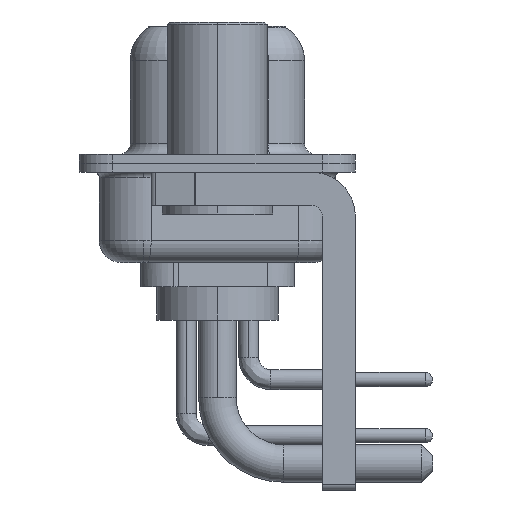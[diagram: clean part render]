
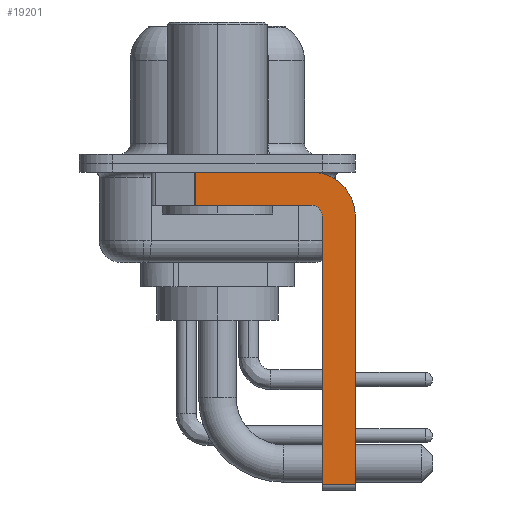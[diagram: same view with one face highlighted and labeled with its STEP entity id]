
A CAD part, left-side view. The second image highlights one B-rep face of the part: STEP entity #19201.
In plain terms, the highlighted planar face has unit normal (-1, 0, 0).
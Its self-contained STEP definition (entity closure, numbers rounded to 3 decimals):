
#447 = ORIENTED_EDGE ( 'NONE', *, *, #19779, .F. ) ;
#1129 = ORIENTED_EDGE ( 'NONE', *, *, #11732, .F. ) ;
#1615 = VERTEX_POINT ( 'NONE', #15081 ) ;
#2427 = CARTESIAN_POINT ( 'NONE',  ( -2.9, -6.25, -2.4 ) ) ;
#2546 = ORIENTED_EDGE ( 'NONE', *, *, #19174, .F. ) ;
#2817 = VERTEX_POINT ( 'NONE', #10769 ) ;
#2862 = CARTESIAN_POINT ( 'NONE',  ( -2.9, -4.25, -2.4 ) ) ;
#3093 = LINE ( 'NONE', #10649, #10733 ) ;
#3225 = DIRECTION ( 'NONE',  ( -1., 0., 0. ) ) ;
#3245 = CARTESIAN_POINT ( 'NONE',  ( -2.9, -6.25, -14.55 ) ) ;
#3899 = LINE ( 'NONE', #17183, #10660 ) ;
#4095 = LINE ( 'NONE', #12005, #23969 ) ;
#4127 = AXIS2_PLACEMENT_3D ( 'NONE', #22752, #5484, #19265 ) ;
#4213 = DIRECTION ( 'NONE',  ( 0., 0., 1. ) ) ;
#4523 = CARTESIAN_POINT ( 'NONE',  ( -2.9, -4.25, -0.4 ) ) ;
#4840 = ORIENTED_EDGE ( 'NONE', *, *, #5111, .F. ) ;
#4882 = ORIENTED_EDGE ( 'NONE', *, *, #15754, .T. ) ;
#5111 = EDGE_CURVE ( 'NONE', #7124, #20126, #13073, .T. ) ;
#5203 = CARTESIAN_POINT ( 'NONE',  ( -2.9, -4.25, -1.9 ) ) ;
#5484 = DIRECTION ( 'NONE',  ( 1., 0., 0. ) ) ;
#5580 = LINE ( 'NONE', #5203, #17742 ) ;
#6432 = EDGE_CURVE ( 'NONE', #2817, #1615, #10281, .T. ) ;
#6849 = ORIENTED_EDGE ( 'NONE', *, *, #19059, .T. ) ;
#7124 = VERTEX_POINT ( 'NONE', #4523 ) ;
#7460 = DIRECTION ( 'NONE',  ( 0., 0., -1. ) ) ;
#7976 = ORIENTED_EDGE ( 'NONE', *, *, #6432, .F. ) ;
#9322 = CARTESIAN_POINT ( 'NONE',  ( -2.9, -6.25, -2.4 ) ) ;
#9692 = LINE ( 'NONE', #9322, #15206 ) ;
#9951 = CARTESIAN_POINT ( 'NONE',  ( -2.9, -4.75, -14.55 ) ) ;
#10281 = CIRCLE ( 'NONE', #20623, 0.5 ) ;
#10412 = DIRECTION ( 'NONE',  ( 0., 0., 1. ) ) ;
#10649 = CARTESIAN_POINT ( 'NONE',  ( -2.9, 3., -0.4 ) ) ;
#10660 = VECTOR ( 'NONE', #15302, 1000. ) ;
#10733 = VECTOR ( 'NONE', #11259, 1000. ) ;
#10769 = CARTESIAN_POINT ( 'NONE',  ( -2.9, -4.75, -2.4 ) ) ;
#11234 = VERTEX_POINT ( 'NONE', #3245 ) ;
#11259 = DIRECTION ( 'NONE',  ( 0., -1., 0. ) ) ;
#11595 = VERTEX_POINT ( 'NONE', #14501 ) ;
#11732 = EDGE_CURVE ( 'NONE', #1615, #11595, #5580, .T. ) ;
#12005 = CARTESIAN_POINT ( 'NONE',  ( -2.9, -4.75, -14.8 ) ) ;
#12376 = CARTESIAN_POINT ( 'NONE',  ( -2.9, -4.25, -2.4 ) ) ;
#12495 = DIRECTION ( 'NONE',  ( 1., 0., 0. ) ) ;
#12826 = VECTOR ( 'NONE', #18406, 1000. ) ;
#12889 = DIRECTION ( 'NONE',  ( 0., 1., 0. ) ) ;
#13073 = CIRCLE ( 'NONE', #18640, 2. ) ;
#14042 = VERTEX_POINT ( 'NONE', #18023 ) ;
#14471 = EDGE_LOOP ( 'NONE', ( #15629, #4882, #1129, #7976, #447, #6849, #2546, #4840 ) ) ;
#14501 = CARTESIAN_POINT ( 'NONE',  ( -2.9, 0.978, -1.9 ) ) ;
#14803 = EDGE_CURVE ( 'NONE', #14042, #7124, #3093, .T. ) ;
#15081 = CARTESIAN_POINT ( 'NONE',  ( -2.9, -4.25, -1.9 ) ) ;
#15206 = VECTOR ( 'NONE', #7460, 1000. ) ;
#15302 = DIRECTION ( 'NONE',  ( 0., 0., -1. ) ) ;
#15629 = ORIENTED_EDGE ( 'NONE', *, *, #14803, .F. ) ;
#15754 = EDGE_CURVE ( 'NONE', #14042, #11595, #3899, .T. ) ;
#17035 = PLANE ( 'NONE',  #4127 ) ;
#17166 = FACE_OUTER_BOUND ( 'NONE', #14471, .T. ) ;
#17183 = CARTESIAN_POINT ( 'NONE',  ( -2.9, 0.978, -1.9 ) ) ;
#17742 = VECTOR ( 'NONE', #12889, 1000. ) ;
#18023 = CARTESIAN_POINT ( 'NONE',  ( -2.9, 0.978, -0.4 ) ) ;
#18236 = DIRECTION ( 'NONE',  ( 0., 0., -1. ) ) ;
#18406 = DIRECTION ( 'NONE',  ( 0., -1., 0. ) ) ;
#18640 = AXIS2_PLACEMENT_3D ( 'NONE', #12376, #12495, #18236 ) ;
#19059 = EDGE_CURVE ( 'NONE', #20873, #11234, #23872, .T. ) ;
#19174 = EDGE_CURVE ( 'NONE', #20126, #11234, #9692, .T. ) ;
#19201 = ADVANCED_FACE ( 'NONE', ( #17166 ), #17035, .F. ) ;
#19265 = DIRECTION ( 'NONE',  ( 0., 0., -1. ) ) ;
#19779 = EDGE_CURVE ( 'NONE', #20873, #2817, #4095, .T. ) ;
#20126 = VERTEX_POINT ( 'NONE', #2427 ) ;
#20623 = AXIS2_PLACEMENT_3D ( 'NONE', #2862, #3225, #10412 ) ;
#20873 = VERTEX_POINT ( 'NONE', #9951 ) ;
#22752 = CARTESIAN_POINT ( 'NONE',  ( -2.9, -4.25, -2.4 ) ) ;
#23872 = LINE ( 'NONE', #24112, #12826 ) ;
#23969 = VECTOR ( 'NONE', #4213, 1000. ) ;
#24112 = CARTESIAN_POINT ( 'NONE',  ( -2.9, -4.25, -14.55 ) ) ;
